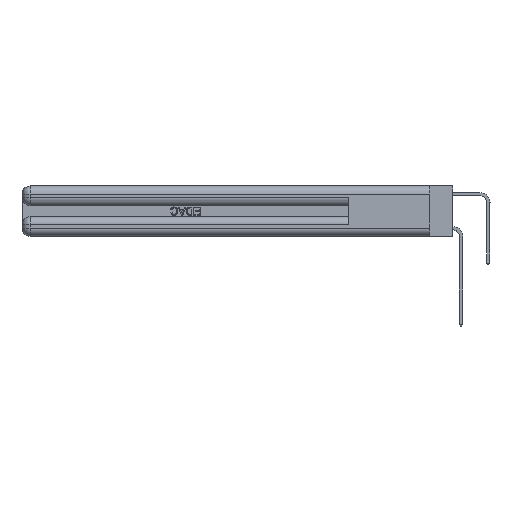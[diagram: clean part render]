
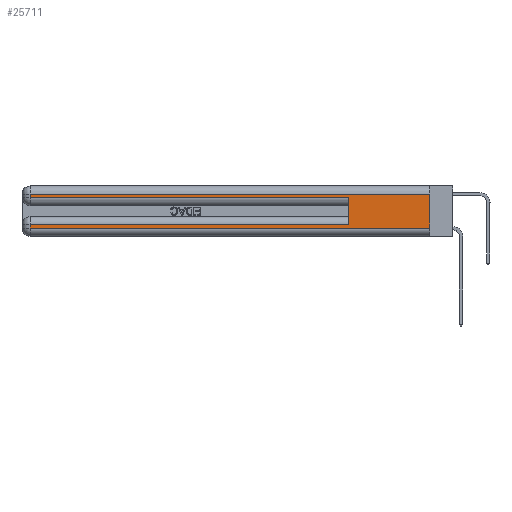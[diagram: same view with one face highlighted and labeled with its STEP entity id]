
A CAD part, left-side view. The second image highlights one B-rep face of the part: STEP entity #25711.
In plain terms, the highlighted planar face has unit normal (-1, 0, 0).
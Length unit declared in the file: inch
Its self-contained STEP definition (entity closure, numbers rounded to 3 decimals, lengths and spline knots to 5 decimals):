
#55 = CARTESIAN_POINT ( 'NONE',  ( 0., 0., 0.085 ) ) ;
#135 = ORIENTED_EDGE ( 'NONE', *, *, #25931, .T. ) ;
#824 = ORIENTED_EDGE ( 'NONE', *, *, #30618, .T. ) ;
#1064 = VECTOR ( 'NONE', #28186, 39.37008 ) ;
#1513 = CARTESIAN_POINT ( 'NONE',  ( 0., 0., 0.06 ) ) ;
#1833 = CARTESIAN_POINT ( 'NONE',  ( 0., 2.94, 0.085 ) ) ;
#2173 = LINE ( 'NONE', #32920, #15331 ) ;
#2507 = CARTESIAN_POINT ( 'NONE',  ( 0., 0.6, 0.085 ) ) ;
#3830 = FACE_OUTER_BOUND ( 'NONE', #25740, .T. ) ;
#3896 = ORIENTED_EDGE ( 'NONE', *, *, #13115, .F. ) ;
#4627 = ORIENTED_EDGE ( 'NONE', *, *, #21238, .T. ) ;
#5193 = CARTESIAN_POINT ( 'NONE',  ( 0., 0., 0.31 ) ) ;
#6955 = PLANE ( 'NONE',  #10783 ) ;
#7486 = LINE ( 'NONE', #31790, #14908 ) ;
#8029 = VECTOR ( 'NONE', #22438, 39.37008 ) ;
#8867 = LINE ( 'NONE', #33610, #1064 ) ;
#10634 = DIRECTION ( 'NONE',  ( 0., -1., 0. ) ) ;
#10715 = CARTESIAN_POINT ( 'NONE',  ( 0., 0.6, 0.145 ) ) ;
#10783 = AXIS2_PLACEMENT_3D ( 'NONE', #14659, #25559, #25331 ) ;
#12196 = CARTESIAN_POINT ( 'NONE',  ( 0., 2.94, 0.37 ) ) ;
#13115 = EDGE_CURVE ( 'NONE', #25260, #24798, #17504, .T. ) ;
#13548 = ORIENTED_EDGE ( 'NONE', *, *, #18521, .T. ) ;
#14659 = CARTESIAN_POINT ( 'NONE',  ( 0., 0., 0.37 ) ) ;
#14740 = VERTEX_POINT ( 'NONE', #19143 ) ;
#14908 = VECTOR ( 'NONE', #10634, 39.37008 ) ;
#15331 = VECTOR ( 'NONE', #19800, 39.37008 ) ;
#15335 = VECTOR ( 'NONE', #21405, 39.37008 ) ;
#15675 = VECTOR ( 'NONE', #31473, 39.37008 ) ;
#15721 = EDGE_CURVE ( 'NONE', #34007, #28931, #2173, .T. ) ;
#17226 = CARTESIAN_POINT ( 'NONE',  ( 0., 0., 0.31 ) ) ;
#17321 = VECTOR ( 'NONE', #31546, 39.37008 ) ;
#17504 = LINE ( 'NONE', #10715, #8029 ) ;
#18521 = EDGE_CURVE ( 'NONE', #14740, #28931, #8867, .T. ) ;
#19070 = CARTESIAN_POINT ( 'NONE',  ( 0., 2.94, 0.31 ) ) ;
#19143 = CARTESIAN_POINT ( 'NONE',  ( 0., 2.94, 0.06 ) ) ;
#19800 = DIRECTION ( 'NONE',  ( 0., 0., -1. ) ) ;
#20744 = CARTESIAN_POINT ( 'NONE',  ( 0., 2.94, 0.37 ) ) ;
#21238 = EDGE_CURVE ( 'NONE', #29224, #24628, #22663, .T. ) ;
#21241 = CARTESIAN_POINT ( 'NONE',  ( 0., 0.6, 0.285 ) ) ;
#21405 = DIRECTION ( 'NONE',  ( 0., 1., 0. ) ) ;
#22313 = LINE ( 'NONE', #55, #15335 ) ;
#22438 = DIRECTION ( 'NONE',  ( 0., 0., 1. ) ) ;
#22663 = LINE ( 'NONE', #20744, #15675 ) ;
#23322 = CARTESIAN_POINT ( 'NONE',  ( 0., 2.94, 0.285 ) ) ;
#23974 = VECTOR ( 'NONE', #28020, 39.37008 ) ;
#24410 = LINE ( 'NONE', #12196, #23974 ) ;
#24628 = VERTEX_POINT ( 'NONE', #23322 ) ;
#24798 = VERTEX_POINT ( 'NONE', #21241 ) ;
#24976 = EDGE_CURVE ( 'NONE', #32986, #14740, #24410, .T. ) ;
#25260 = VERTEX_POINT ( 'NONE', #2507 ) ;
#25331 = DIRECTION ( 'NONE',  ( 0., 0., -1. ) ) ;
#25559 = DIRECTION ( 'NONE',  ( 1., 0., 0. ) ) ;
#25711 = ADVANCED_FACE ( 'NONE', ( #3830 ), #6955, .F. ) ;
#25740 = EDGE_LOOP ( 'NONE', ( #30257, #824, #4627, #33684, #3896, #135, #26478, #13548 ) ) ;
#25931 = EDGE_CURVE ( 'NONE', #25260, #32986, #22313, .T. ) ;
#26044 = EDGE_CURVE ( 'NONE', #24628, #24798, #7486, .T. ) ;
#26478 = ORIENTED_EDGE ( 'NONE', *, *, #24976, .T. ) ;
#28020 = DIRECTION ( 'NONE',  ( 0., 0., -1. ) ) ;
#28186 = DIRECTION ( 'NONE',  ( 0., -1., 0. ) ) ;
#28931 = VERTEX_POINT ( 'NONE', #1513 ) ;
#29224 = VERTEX_POINT ( 'NONE', #19070 ) ;
#30116 = LINE ( 'NONE', #5193, #17321 ) ;
#30257 = ORIENTED_EDGE ( 'NONE', *, *, #15721, .F. ) ;
#30618 = EDGE_CURVE ( 'NONE', #34007, #29224, #30116, .T. ) ;
#31473 = DIRECTION ( 'NONE',  ( 0., 0., -1. ) ) ;
#31546 = DIRECTION ( 'NONE',  ( 0., 1., 0. ) ) ;
#31790 = CARTESIAN_POINT ( 'NONE',  ( 0., 0., 0.285 ) ) ;
#32920 = CARTESIAN_POINT ( 'NONE',  ( 0., 0., 0.37 ) ) ;
#32986 = VERTEX_POINT ( 'NONE', #1833 ) ;
#33610 = CARTESIAN_POINT ( 'NONE',  ( 0., 0., 0.06 ) ) ;
#33684 = ORIENTED_EDGE ( 'NONE', *, *, #26044, .T. ) ;
#34007 = VERTEX_POINT ( 'NONE', #17226 ) ;
